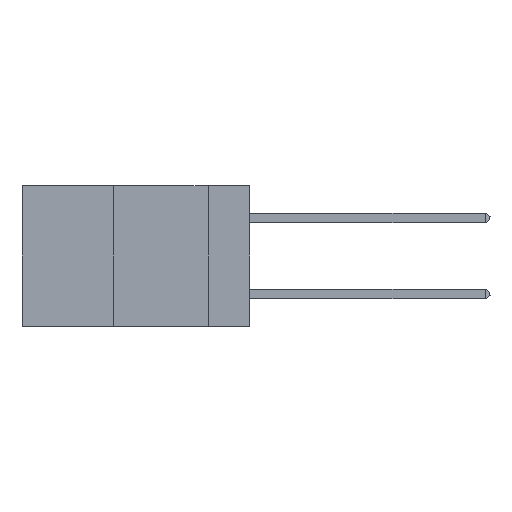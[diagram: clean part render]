
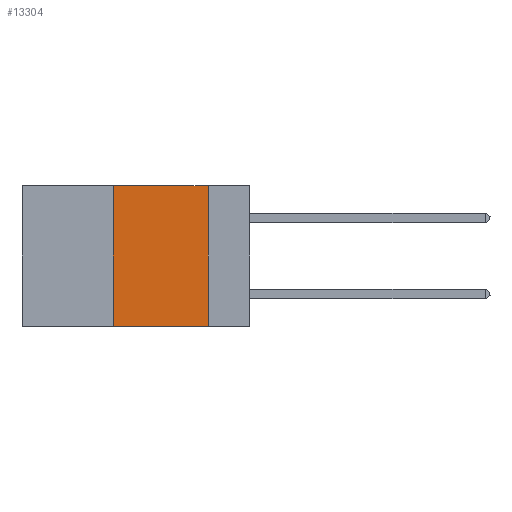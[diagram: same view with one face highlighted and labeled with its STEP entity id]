
A CAD part, left-side view. The second image highlights one B-rep face of the part: STEP entity #13304.
In plain terms, the highlighted planar face has unit normal (-1, 0, 0).
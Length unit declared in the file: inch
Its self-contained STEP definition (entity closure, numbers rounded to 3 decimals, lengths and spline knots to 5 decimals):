
#9 = CARTESIAN_POINT ( 'NONE',  ( 0., 0.36, -0.37 ) ) ;
#947 = LINE ( 'NONE', #29675, #33681 ) ;
#1040 = ORIENTED_EDGE ( 'NONE', *, *, #27803, .F. ) ;
#2176 = LINE ( 'NONE', #26612, #10637 ) ;
#4850 = CARTESIAN_POINT ( 'NONE',  ( 0., 0.11, 0. ) ) ;
#5029 = VERTEX_POINT ( 'NONE', #4850 ) ;
#8031 = DIRECTION ( 'NONE',  ( 0., 0., -1. ) ) ;
#10131 = EDGE_CURVE ( 'NONE', #43533, #36689, #10668, .T. ) ;
#10637 = VECTOR ( 'NONE', #19479, 39.37008 ) ;
#10668 = LINE ( 'NONE', #26122, #24879 ) ;
#11433 = ORIENTED_EDGE ( 'NONE', *, *, #42750, .F. ) ;
#13304 = ADVANCED_FACE ( 'NONE', ( #31857 ), #40767, .F. ) ;
#13964 = DIRECTION ( 'NONE',  ( 0., -1., 0. ) ) ;
#15049 = DIRECTION ( 'NONE',  ( 0., -1., 0. ) ) ;
#15821 = DIRECTION ( 'NONE',  ( 1., 0., 0. ) ) ;
#19301 = DIRECTION ( 'NONE',  ( 0., 0., -1. ) ) ;
#19479 = DIRECTION ( 'NONE',  ( 0., 0., 1. ) ) ;
#19743 = VECTOR ( 'NONE', #13964, 39.37008 ) ;
#22082 = CARTESIAN_POINT ( 'NONE',  ( 0., 0.36, 0. ) ) ;
#22131 = ORIENTED_EDGE ( 'NONE', *, *, #37780, .F. ) ;
#24879 = VECTOR ( 'NONE', #15049, 39.37008 ) ;
#26122 = CARTESIAN_POINT ( 'NONE',  ( 0., 0.6, -0.37 ) ) ;
#26273 = VERTEX_POINT ( 'NONE', #22082 ) ;
#26612 = CARTESIAN_POINT ( 'NONE',  ( 0., 0.36, 0. ) ) ;
#27803 = EDGE_CURVE ( 'NONE', #5029, #36689, #947, .T. ) ;
#29381 = LINE ( 'NONE', #45553, #19743 ) ;
#29675 = CARTESIAN_POINT ( 'NONE',  ( 0., 0.11, 0. ) ) ;
#29864 = AXIS2_PLACEMENT_3D ( 'NONE', #40471, #15821, #19301 ) ;
#31857 = FACE_OUTER_BOUND ( 'NONE', #43023, .T. ) ;
#32282 = CARTESIAN_POINT ( 'NONE',  ( 0., 0.11, -0.37 ) ) ;
#33681 = VECTOR ( 'NONE', #8031, 39.37008 ) ;
#36689 = VERTEX_POINT ( 'NONE', #32282 ) ;
#37780 = EDGE_CURVE ( 'NONE', #26273, #5029, #29381, .T. ) ;
#40471 = CARTESIAN_POINT ( 'NONE',  ( 0., 0.6, 0. ) ) ;
#40767 = PLANE ( 'NONE',  #29864 ) ;
#42750 = EDGE_CURVE ( 'NONE', #43533, #26273, #2176, .T. ) ;
#43023 = EDGE_LOOP ( 'NONE', ( #1040, #22131, #11433, #45581 ) ) ;
#43533 = VERTEX_POINT ( 'NONE', #9 ) ;
#45553 = CARTESIAN_POINT ( 'NONE',  ( 0., 0.6, 0. ) ) ;
#45581 = ORIENTED_EDGE ( 'NONE', *, *, #10131, .T. ) ;
